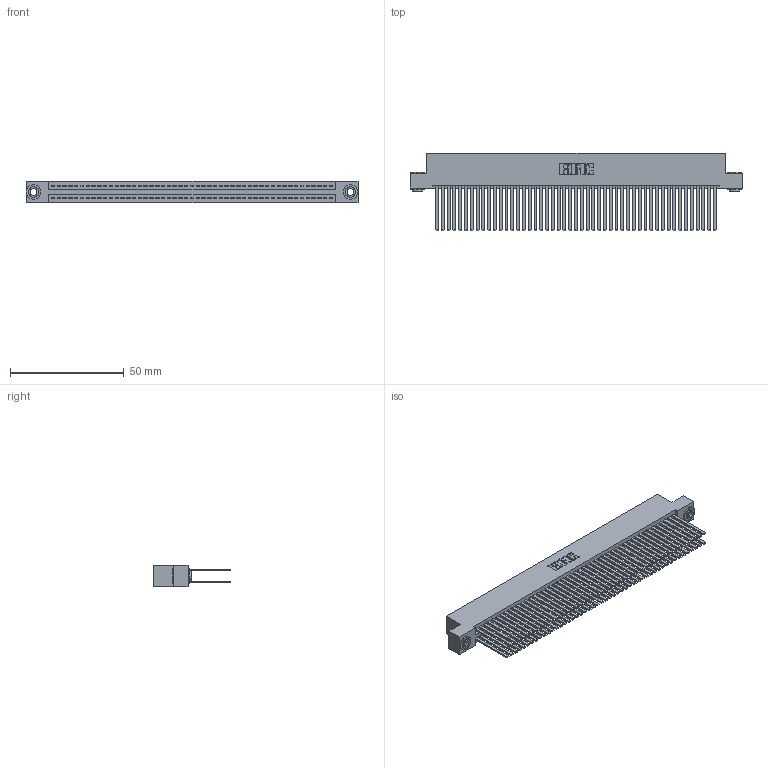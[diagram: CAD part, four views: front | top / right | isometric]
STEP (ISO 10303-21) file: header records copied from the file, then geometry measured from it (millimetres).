
FILE_DESCRIPTION (( 'STEP AP203' ), '1' );
FILE_NAME ('345-098-544-203.STEP', '2019-11-02T12:03:57', ( '' ), ( '' ), 'SwSTEP 2.0', 'SolidWorks 2016', '' );
FILE_SCHEMA (( 'CONFIG_CONTROL_DESIGN' ));
Length unit declared in the file: inch
Products named in the file (4): 345-250-002_345-250-002-102; 345 Part_Flush Mounting Lugs - 0.156 Dia-TH; 345-098-544-203; 345-292-001_345-293-144
Assembly tree (101 placements, depth 2):
  345-098-544-203
    345 Part_Flush Mounting Lugs - 0.156 Dia-TH
    345-292-001_345-293-144  x98
    345-250-002_345-250-002-102  x2
Bounding box: 145.67 x 33.96 x 9.4 mm (x, y, z)
Volume: 15608.6 mm3; surface area: 27439 mm2
Topology: 101 solids, 101 shells, 4476 faces, 13255 edges, 8702 vertices
Faces by surface type: plane 2932, cylinder 1536, cone 8
Entity records: 37970 total; most frequent: CARTESIAN_POINT 6331, ORIENTED_EDGE 6258, DIRECTION 5603, EDGE_CURVE 3129, VECTOR 2781, LINE 2781, VERTEX_POINT 2082, AXIS2_PLACEMENT_3D 1411
